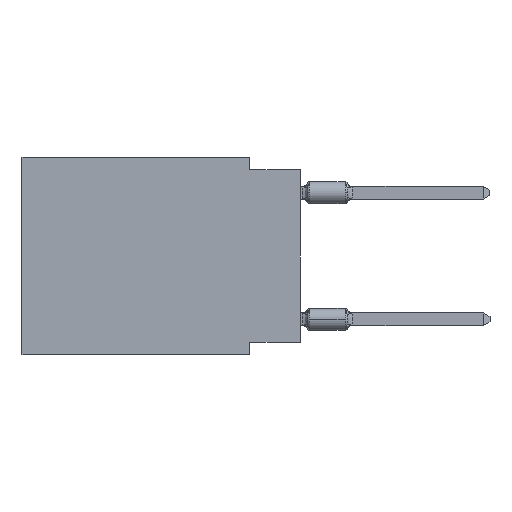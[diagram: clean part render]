
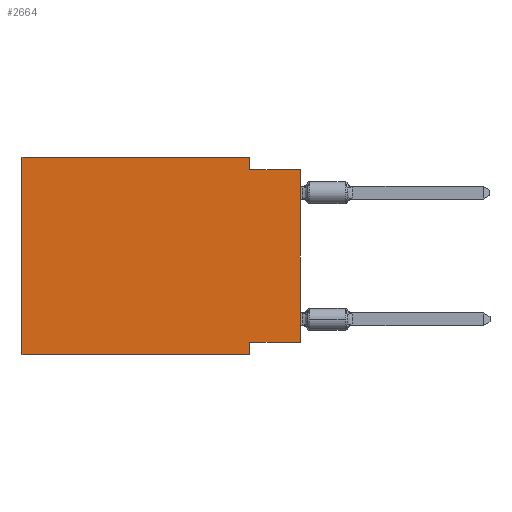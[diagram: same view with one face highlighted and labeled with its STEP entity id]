
A CAD part, left-side view. The second image highlights one B-rep face of the part: STEP entity #2664.
In plain terms, the highlighted planar face has unit normal (-1, 0, 0).
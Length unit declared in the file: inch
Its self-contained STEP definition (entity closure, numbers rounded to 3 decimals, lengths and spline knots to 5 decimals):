
#232 = LINE ( 'NONE', #6984, #486 ) ;
#257 = LINE ( 'NONE', #4690, #1484 ) ;
#486 = VECTOR ( 'NONE', #11442, 39.37008 ) ;
#552 = EDGE_CURVE ( 'NONE', #13205, #12386, #232, .T. ) ;
#685 = VERTEX_POINT ( 'NONE', #2697 ) ;
#747 = CARTESIAN_POINT ( 'NONE',  ( 0., 0.55, -0.39 ) ) ;
#764 = CARTESIAN_POINT ( 'NONE',  ( 0., 0.55, 0. ) ) ;
#826 = VERTEX_POINT ( 'NONE', #3124 ) ;
#1044 = DIRECTION ( 'NONE',  ( 0., 0., -1. ) ) ;
#1049 = VERTEX_POINT ( 'NONE', #3978 ) ;
#1053 = VECTOR ( 'NONE', #1044, 39.37008 ) ;
#1138 = CARTESIAN_POINT ( 'NONE',  ( 0., 0.1, 0. ) ) ;
#1160 = EDGE_LOOP ( 'NONE', ( #13474, #6772, #2363, #4519, #4332, #11617, #4063, #7395 ) ) ;
#1411 = FACE_OUTER_BOUND ( 'NONE', #1160, .T. ) ;
#1484 = VECTOR ( 'NONE', #9131, 39.37008 ) ;
#2110 = VECTOR ( 'NONE', #13708, 39.37008 ) ;
#2185 = LINE ( 'NONE', #12220, #11280 ) ;
#2306 = EDGE_CURVE ( 'NONE', #826, #1049, #257, .T. ) ;
#2363 = ORIENTED_EDGE ( 'NONE', *, *, #552, .F. ) ;
#2460 = VERTEX_POINT ( 'NONE', #764 ) ;
#2578 = LINE ( 'NONE', #12479, #2110 ) ;
#2664 = ADVANCED_FACE ( 'NONE', ( #1411 ), #8902, .F. ) ;
#2697 = CARTESIAN_POINT ( 'NONE',  ( 0., 0.55, -0.39 ) ) ;
#3124 = CARTESIAN_POINT ( 'NONE',  ( 0., 0., -0.365 ) ) ;
#3340 = VERTEX_POINT ( 'NONE', #6253 ) ;
#3437 = CARTESIAN_POINT ( 'NONE',  ( 0., 0.55, 0. ) ) ;
#3746 = DIRECTION ( 'NONE',  ( 0., -1., 0. ) ) ;
#3978 = CARTESIAN_POINT ( 'NONE',  ( 0., 0.1, -0.365 ) ) ;
#4002 = EDGE_CURVE ( 'NONE', #1049, #9231, #6273, .T. ) ;
#4063 = ORIENTED_EDGE ( 'NONE', *, *, #4002, .F. ) ;
#4066 = CARTESIAN_POINT ( 'NONE',  ( 0., 0.1, -0.025 ) ) ;
#4294 = DIRECTION ( 'NONE',  ( 0., 0., 1. ) ) ;
#4332 = ORIENTED_EDGE ( 'NONE', *, *, #4559, .F. ) ;
#4456 = EDGE_CURVE ( 'NONE', #826, #3340, #10776, .T. ) ;
#4504 = DIRECTION ( 'NONE',  ( 0., 0., 1. ) ) ;
#4519 = ORIENTED_EDGE ( 'NONE', *, *, #10216, .F. ) ;
#4559 = EDGE_CURVE ( 'NONE', #685, #2460, #2185, .T. ) ;
#4690 = CARTESIAN_POINT ( 'NONE',  ( 0., 0., -0.365 ) ) ;
#6253 = CARTESIAN_POINT ( 'NONE',  ( 0., 0., -0.025 ) ) ;
#6273 = LINE ( 'NONE', #7504, #1053 ) ;
#6473 = CARTESIAN_POINT ( 'NONE',  ( 0., 0., 0. ) ) ;
#6619 = VECTOR ( 'NONE', #4294, 39.37008 ) ;
#6772 = ORIENTED_EDGE ( 'NONE', *, *, #14132, .F. ) ;
#6984 = CARTESIAN_POINT ( 'NONE',  ( 0., 0.1, 0. ) ) ;
#7350 = LINE ( 'NONE', #747, #9340 ) ;
#7395 = ORIENTED_EDGE ( 'NONE', *, *, #2306, .F. ) ;
#7504 = CARTESIAN_POINT ( 'NONE',  ( 0., 0.1, -0.39 ) ) ;
#7805 = DIRECTION ( 'NONE',  ( 0., 0., -1. ) ) ;
#8202 = AXIS2_PLACEMENT_3D ( 'NONE', #3437, #13340, #7805 ) ;
#8884 = DIRECTION ( 'NONE',  ( 0., -1., 0. ) ) ;
#8902 = PLANE ( 'NONE',  #8202 ) ;
#9131 = DIRECTION ( 'NONE',  ( 0., 1., 0. ) ) ;
#9231 = VERTEX_POINT ( 'NONE', #12256 ) ;
#9340 = VECTOR ( 'NONE', #3746, 39.37008 ) ;
#10049 = LINE ( 'NONE', #13257, #11448 ) ;
#10216 = EDGE_CURVE ( 'NONE', #2460, #13205, #2578, .T. ) ;
#10776 = LINE ( 'NONE', #6473, #6619 ) ;
#11280 = VECTOR ( 'NONE', #4504, 39.37008 ) ;
#11442 = DIRECTION ( 'NONE',  ( 0., 0., -1. ) ) ;
#11448 = VECTOR ( 'NONE', #8884, 39.37008 ) ;
#11617 = ORIENTED_EDGE ( 'NONE', *, *, #12027, .T. ) ;
#12027 = EDGE_CURVE ( 'NONE', #685, #9231, #7350, .T. ) ;
#12220 = CARTESIAN_POINT ( 'NONE',  ( 0., 0.55, 0. ) ) ;
#12256 = CARTESIAN_POINT ( 'NONE',  ( 0., 0.1, -0.39 ) ) ;
#12386 = VERTEX_POINT ( 'NONE', #4066 ) ;
#12479 = CARTESIAN_POINT ( 'NONE',  ( 0., 0.55, 0. ) ) ;
#13205 = VERTEX_POINT ( 'NONE', #1138 ) ;
#13257 = CARTESIAN_POINT ( 'NONE',  ( 0., 0., -0.025 ) ) ;
#13340 = DIRECTION ( 'NONE',  ( 1., 0., 0. ) ) ;
#13474 = ORIENTED_EDGE ( 'NONE', *, *, #4456, .T. ) ;
#13708 = DIRECTION ( 'NONE',  ( 0., -1., 0. ) ) ;
#14132 = EDGE_CURVE ( 'NONE', #12386, #3340, #10049, .T. ) ;
